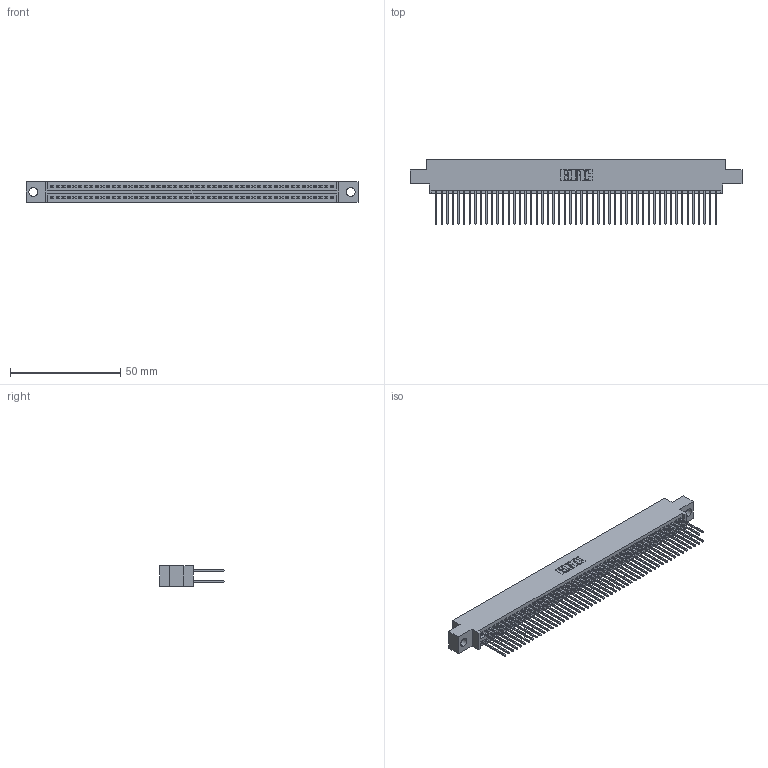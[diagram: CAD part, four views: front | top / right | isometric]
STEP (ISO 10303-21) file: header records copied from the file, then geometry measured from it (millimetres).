
FILE_DESCRIPTION (( 'STEP AP203' ), '1' );
FILE_NAME ('345-102-540-804.STEP', '2018-10-05T19:47:33', ( '' ), ( '' ), 'SwSTEP 2.0', 'SolidWorks 2016', '' );
FILE_SCHEMA (( 'CONFIG_CONTROL_DESIGN' ));
Length unit declared in the file: inch
Products named in the file (3): 345 Part_0.170 Offset - 0.156 Dia-TH; 345-292-001_345-293-140; 345-102-540-804
Assembly tree (103 placements, depth 2):
  345-102-540-804
    345 Part_0.170 Offset - 0.156 Dia-TH
    345-292-001_345-293-140  x102
Bounding box: 150.75 x 29.13 x 9.4 mm (x, y, z)
Volume: 14912.9 mm3; surface area: 23970.7 mm2
Topology: 103 solids, 103 shells, 5230 faces, 15551 edges, 10230 vertices
Faces by surface type: plane 3450, cylinder 1780
Entity records: 38957 total; most frequent: CARTESIAN_POINT 6524, ORIENTED_EDGE 6458, DIRECTION 5741, EDGE_CURVE 3229, VECTOR 2893, LINE 2893, VERTEX_POINT 2150, AXIS2_PLACEMENT_3D 1424
